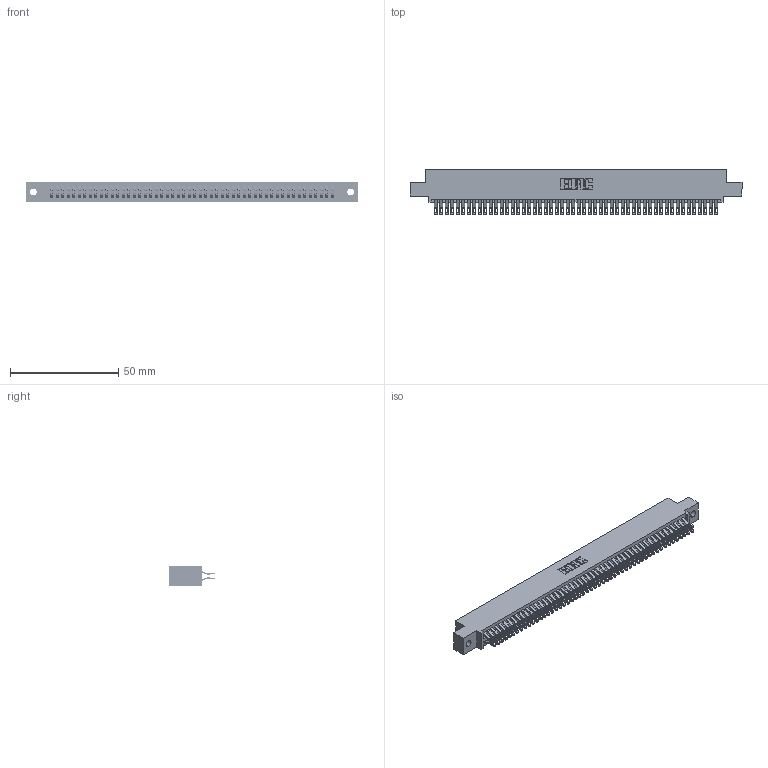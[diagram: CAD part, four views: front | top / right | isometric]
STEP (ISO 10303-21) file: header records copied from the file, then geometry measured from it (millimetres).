
FILE_DESCRIPTION (( 'STEP AP203' ), '1' );
FILE_NAME ('395-104-555-502.STEP', '2018-11-30T13:54:42', ( '' ), ( '' ), 'SwSTEP 2.0', 'SolidWorks 2016', '' );
FILE_SCHEMA (( 'CONFIG_CONTROL_DESIGN' ));
Length unit declared in the file: inch
Products named in the file (3): 345 Part_0.110 Offset - 0.128 Dia; 345-292-001_555 Tail; 395-104-555-502
Assembly tree (105 placements, depth 2):
  395-104-555-502
    345 Part_0.110 Offset - 0.128 Dia
    345-292-001_555 Tail  x104
Bounding box: 153.29 x 21.13 x 9.4 mm (x, y, z)
Volume: 15175.1 mm3; surface area: 23494.3 mm2
Topology: 105 solids, 105 shells, 5954 faces, 18761 edges, 12506 vertices
Faces by surface type: plane 3308, cylinder 2646
Entity records: 39915 total; most frequent: CARTESIAN_POINT 6718, ORIENTED_EDGE 6622, DIRECTION 5879, EDGE_CURVE 3311, VECTOR 2951, LINE 2951, VERTEX_POINT 2206, AXIS2_PLACEMENT_3D 1464
